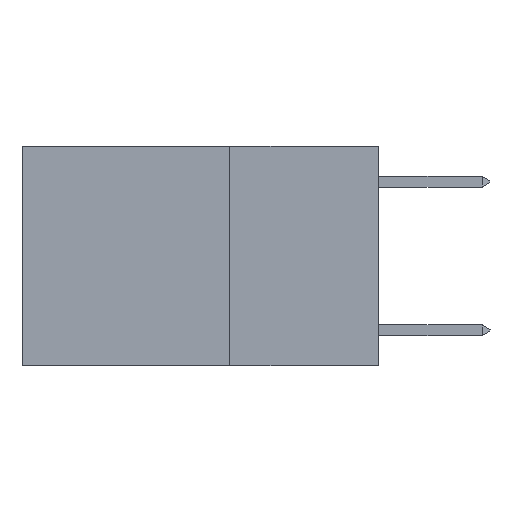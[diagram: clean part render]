
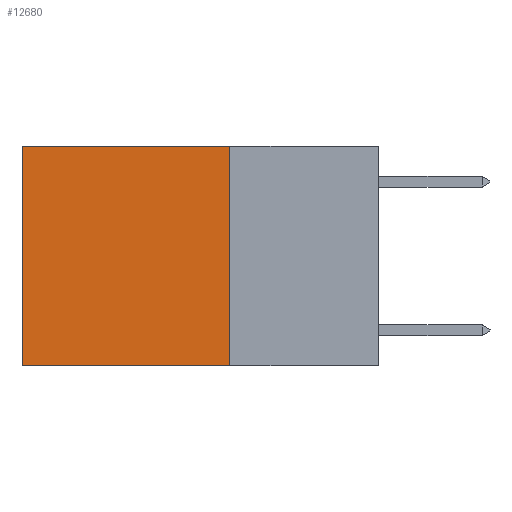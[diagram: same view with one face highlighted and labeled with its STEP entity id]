
A CAD part, left-side view. The second image highlights one B-rep face of the part: STEP entity #12680.
In plain terms, the highlighted planar face has unit normal (-1, 0, 0).
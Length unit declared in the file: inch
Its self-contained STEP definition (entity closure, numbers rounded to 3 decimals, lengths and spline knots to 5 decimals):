
#1547 = EDGE_CURVE ( 'NONE', #22186, #21094, #9512, .T. ) ;
#3910 = AXIS2_PLACEMENT_3D ( 'NONE', #13758, #13117, #12976 ) ;
#6183 = DIRECTION ( 'NONE',  ( 0., 0., -1. ) ) ;
#6482 = CARTESIAN_POINT ( 'NONE',  ( 0.2625, 0.25, 0. ) ) ;
#6585 = CARTESIAN_POINT ( 'NONE',  ( 0.2625, 0.25, 0. ) ) ;
#6846 = VECTOR ( 'NONE', #7462, 39.37008 ) ;
#6869 = LINE ( 'NONE', #8172, #6846 ) ;
#7462 = DIRECTION ( 'NONE',  ( 0., 1., 0. ) ) ;
#7709 = EDGE_CURVE ( 'NONE', #8081, #21094, #22370, .T. ) ;
#8081 = VERTEX_POINT ( 'NONE', #11157 ) ;
#8172 = CARTESIAN_POINT ( 'NONE',  ( 0.2625, 0.25, 0. ) ) ;
#9487 = VECTOR ( 'NONE', #12742, 39.37008 ) ;
#9512 = LINE ( 'NONE', #13399, #9487 ) ;
#9756 = CARTESIAN_POINT ( 'NONE',  ( 0.2625, 0.6, -0.37 ) ) ;
#9917 = ORIENTED_EDGE ( 'NONE', *, *, #7709, .F. ) ;
#9931 = ORIENTED_EDGE ( 'NONE', *, *, #9953, .T. ) ;
#9953 = EDGE_CURVE ( 'NONE', #17838, #22186, #6869, .T. ) ;
#10147 = ORIENTED_EDGE ( 'NONE', *, *, #1547, .T. ) ;
#10256 = ORIENTED_EDGE ( 'NONE', *, *, #14616, .F. ) ;
#11157 = CARTESIAN_POINT ( 'NONE',  ( 0.2625, 0.25, -0.37 ) ) ;
#12680 = ADVANCED_FACE ( 'NONE', ( #19211 ), #14737, .F. ) ;
#12742 = DIRECTION ( 'NONE',  ( 0., 0., -1. ) ) ;
#12976 = DIRECTION ( 'NONE',  ( 0., 0., -1. ) ) ;
#13117 = DIRECTION ( 'NONE',  ( 1., 0., 0. ) ) ;
#13399 = CARTESIAN_POINT ( 'NONE',  ( 0.2625, 0.6, 0. ) ) ;
#13758 = CARTESIAN_POINT ( 'NONE',  ( 0.2625, 0.25, 0. ) ) ;
#14616 = EDGE_CURVE ( 'NONE', #17838, #8081, #19445, .T. ) ;
#14737 = PLANE ( 'NONE',  #3910 ) ;
#17381 = DIRECTION ( 'NONE',  ( 0., 1., 0. ) ) ;
#17456 = CARTESIAN_POINT ( 'NONE',  ( 0.2625, 0.25, -0.37 ) ) ;
#17838 = VERTEX_POINT ( 'NONE', #6482 ) ;
#18822 = CARTESIAN_POINT ( 'NONE',  ( 0.2625, 0.6, 0. ) ) ;
#19211 = FACE_OUTER_BOUND ( 'NONE', #20253, .T. ) ;
#19418 = VECTOR ( 'NONE', #6183, 39.37008 ) ;
#19445 = LINE ( 'NONE', #6585, #19418 ) ;
#20253 = EDGE_LOOP ( 'NONE', ( #10147, #9917, #10256, #9931 ) ) ;
#21094 = VERTEX_POINT ( 'NONE', #9756 ) ;
#22186 = VERTEX_POINT ( 'NONE', #18822 ) ;
#22244 = VECTOR ( 'NONE', #17381, 39.37008 ) ;
#22370 = LINE ( 'NONE', #17456, #22244 ) ;
